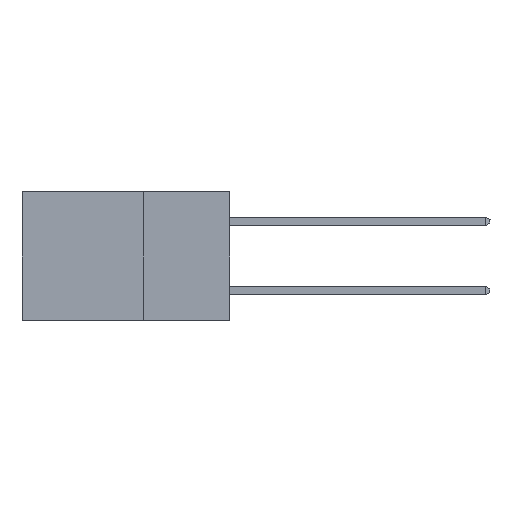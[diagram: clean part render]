
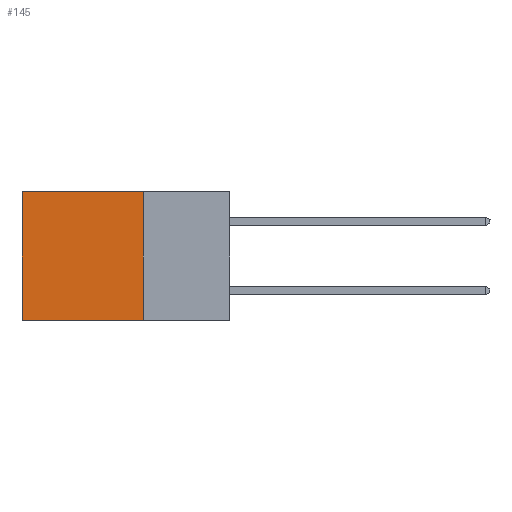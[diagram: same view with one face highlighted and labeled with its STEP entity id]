
A CAD part, left-side view. The second image highlights one B-rep face of the part: STEP entity #145.
In plain terms, the highlighted planar face has unit normal (-1, 0, 0).
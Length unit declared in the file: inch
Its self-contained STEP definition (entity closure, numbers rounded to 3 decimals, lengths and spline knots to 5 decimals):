
#145 = ADVANCED_FACE ( 'NONE', ( #1577 ), #2693, .F. ) ;
#393 = CARTESIAN_POINT ( 'NONE',  ( 0.2615, 0.25, -0.37 ) ) ;
#557 = ORIENTED_EDGE ( 'NONE', *, *, #4632, .F. ) ;
#657 = ORIENTED_EDGE ( 'NONE', *, *, #8014, .F. ) ;
#676 = EDGE_LOOP ( 'NONE', ( #6115, #657, #557, #3901 ) ) ;
#771 = CARTESIAN_POINT ( 'NONE',  ( 0.2615, 0.6, 0. ) ) ;
#1210 = CARTESIAN_POINT ( 'NONE',  ( 0.2615, 0.25, 0. ) ) ;
#1507 = VECTOR ( 'NONE', #10713, 39.37008 ) ;
#1577 = FACE_OUTER_BOUND ( 'NONE', #676, .T. ) ;
#2693 = PLANE ( 'NONE',  #5459 ) ;
#3044 = VECTOR ( 'NONE', #8604, 39.37008 ) ;
#3079 = CARTESIAN_POINT ( 'NONE',  ( 0.2615, 0.25, -0.37 ) ) ;
#3222 = VECTOR ( 'NONE', #10569, 39.37008 ) ;
#3309 = EDGE_CURVE ( 'NONE', #10704, #7794, #6892, .T. ) ;
#3901 = ORIENTED_EDGE ( 'NONE', *, *, #3309, .T. ) ;
#4632 = EDGE_CURVE ( 'NONE', #10704, #6995, #9761, .T. ) ;
#5459 = AXIS2_PLACEMENT_3D ( 'NONE', #9207, #6449, #12085 ) ;
#6001 = DIRECTION ( 'NONE',  ( 0., 1., 0. ) ) ;
#6115 = ORIENTED_EDGE ( 'NONE', *, *, #8468, .T. ) ;
#6449 = DIRECTION ( 'NONE',  ( 1., 0., 0. ) ) ;
#6660 = VECTOR ( 'NONE', #6001, 39.37008 ) ;
#6892 = LINE ( 'NONE', #1210, #3222 ) ;
#6918 = CARTESIAN_POINT ( 'NONE',  ( 0.2615, 0.6, -0.37 ) ) ;
#6932 = LINE ( 'NONE', #393, #6660 ) ;
#6995 = VERTEX_POINT ( 'NONE', #11391 ) ;
#7347 = VERTEX_POINT ( 'NONE', #9340 ) ;
#7794 = VERTEX_POINT ( 'NONE', #771 ) ;
#7838 = LINE ( 'NONE', #6918, #1507 ) ;
#8014 = EDGE_CURVE ( 'NONE', #6995, #7347, #6932, .T. ) ;
#8468 = EDGE_CURVE ( 'NONE', #7794, #7347, #7838, .T. ) ;
#8604 = DIRECTION ( 'NONE',  ( 0., 0., -1. ) ) ;
#9207 = CARTESIAN_POINT ( 'NONE',  ( 0.2615, 0.25, -0.37 ) ) ;
#9340 = CARTESIAN_POINT ( 'NONE',  ( 0.2615, 0.6, -0.37 ) ) ;
#9761 = LINE ( 'NONE', #3079, #3044 ) ;
#10569 = DIRECTION ( 'NONE',  ( 0., 1., 0. ) ) ;
#10704 = VERTEX_POINT ( 'NONE', #11234 ) ;
#10713 = DIRECTION ( 'NONE',  ( 0., 0., -1. ) ) ;
#11234 = CARTESIAN_POINT ( 'NONE',  ( 0.2615, 0.25, 0. ) ) ;
#11391 = CARTESIAN_POINT ( 'NONE',  ( 0.2615, 0.25, -0.37 ) ) ;
#12085 = DIRECTION ( 'NONE',  ( 0., 0., -1. ) ) ;
